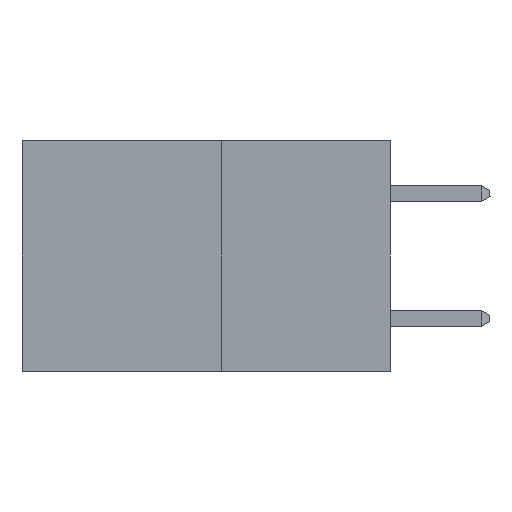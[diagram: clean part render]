
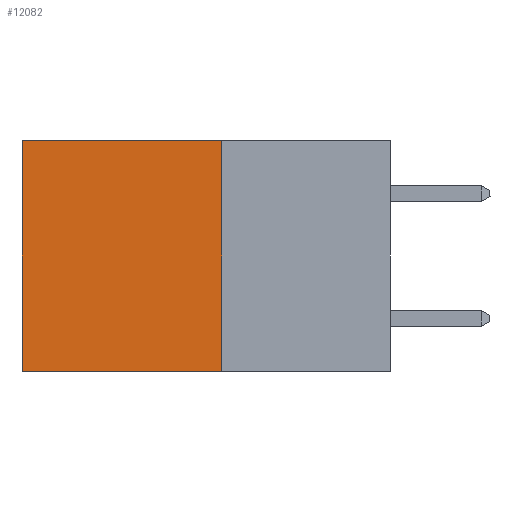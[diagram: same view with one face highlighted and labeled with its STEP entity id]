
A CAD part, left-side view. The second image highlights one B-rep face of the part: STEP entity #12082.
In plain terms, the highlighted planar face has unit normal (-1, 0, 0).
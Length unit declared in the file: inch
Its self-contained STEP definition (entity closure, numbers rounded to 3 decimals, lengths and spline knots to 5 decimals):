
#74 = VECTOR ( 'NONE', #15131, 39.37008 ) ;
#220 = CARTESIAN_POINT ( 'NONE',  ( 0.277, 0.27, -0.37 ) ) ;
#1040 = LINE ( 'NONE', #2522, #4165 ) ;
#1553 = ORIENTED_EDGE ( 'NONE', *, *, #16331, .F. ) ;
#1742 = VERTEX_POINT ( 'NONE', #12946 ) ;
#1749 = CARTESIAN_POINT ( 'NONE',  ( 0.277, 0.27, 0. ) ) ;
#2522 = CARTESIAN_POINT ( 'NONE',  ( 0.277, 0.27, -0.37 ) ) ;
#3328 = CARTESIAN_POINT ( 'NONE',  ( 0.277, 0.27, -0.37 ) ) ;
#3635 = LINE ( 'NONE', #11383, #74 ) ;
#3741 = VERTEX_POINT ( 'NONE', #1749 ) ;
#4165 = VECTOR ( 'NONE', #12960, 39.37008 ) ;
#5149 = EDGE_CURVE ( 'NONE', #3741, #7182, #15945, .T. ) ;
#5544 = DIRECTION ( 'NONE',  ( 0., 0., -1. ) ) ;
#6982 = EDGE_CURVE ( 'NONE', #3741, #15206, #8379, .T. ) ;
#7182 = VERTEX_POINT ( 'NONE', #16622 ) ;
#7333 = CARTESIAN_POINT ( 'NONE',  ( 0.277, 0.27, -0.37 ) ) ;
#7348 = DIRECTION ( 'NONE',  ( 0., 0., -1. ) ) ;
#7666 = DIRECTION ( 'NONE',  ( 0., 1., 0. ) ) ;
#7763 = CARTESIAN_POINT ( 'NONE',  ( 0.277, 0.27, 0. ) ) ;
#8379 = LINE ( 'NONE', #7333, #11847 ) ;
#9715 = VECTOR ( 'NONE', #7666, 39.37008 ) ;
#10207 = AXIS2_PLACEMENT_3D ( 'NONE', #220, #13311, #5544 ) ;
#10660 = EDGE_LOOP ( 'NONE', ( #15318, #1553, #14563, #10851 ) ) ;
#10851 = ORIENTED_EDGE ( 'NONE', *, *, #5149, .T. ) ;
#11383 = CARTESIAN_POINT ( 'NONE',  ( 0.277, 0.59, -0.37 ) ) ;
#11847 = VECTOR ( 'NONE', #7348, 39.37008 ) ;
#12082 = ADVANCED_FACE ( 'NONE', ( #16591 ), #15700, .F. ) ;
#12274 = EDGE_CURVE ( 'NONE', #7182, #1742, #3635, .T. ) ;
#12946 = CARTESIAN_POINT ( 'NONE',  ( 0.277, 0.59, -0.37 ) ) ;
#12960 = DIRECTION ( 'NONE',  ( 0., 1., 0. ) ) ;
#13311 = DIRECTION ( 'NONE',  ( 1., 0., 0. ) ) ;
#14563 = ORIENTED_EDGE ( 'NONE', *, *, #6982, .F. ) ;
#15131 = DIRECTION ( 'NONE',  ( 0., 0., -1. ) ) ;
#15206 = VERTEX_POINT ( 'NONE', #3328 ) ;
#15318 = ORIENTED_EDGE ( 'NONE', *, *, #12274, .T. ) ;
#15700 = PLANE ( 'NONE',  #10207 ) ;
#15945 = LINE ( 'NONE', #7763, #9715 ) ;
#16331 = EDGE_CURVE ( 'NONE', #15206, #1742, #1040, .T. ) ;
#16591 = FACE_OUTER_BOUND ( 'NONE', #10660, .T. ) ;
#16622 = CARTESIAN_POINT ( 'NONE',  ( 0.277, 0.59, 0. ) ) ;
